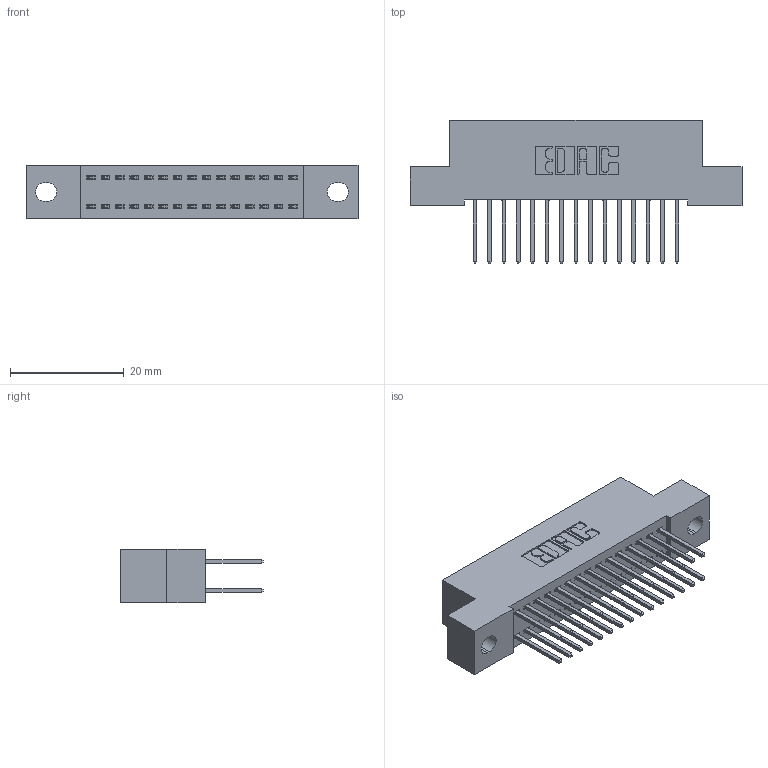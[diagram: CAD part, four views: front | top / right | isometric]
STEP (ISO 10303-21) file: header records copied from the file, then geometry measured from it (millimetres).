
FILE_DESCRIPTION (( 'STEP AP203' ), '1' );
FILE_NAME ('392-030-523-202.STEP', '2018-08-15T22:16:20', ( '' ), ( '' ), 'SwSTEP 2.0', 'SolidWorks 2016', '' );
FILE_SCHEMA (( 'CONFIG_CONTROL_DESIGN' ));
Length unit declared in the file: inch
Products named in the file (3): 342 Part_.128 Slot; 345-292-001_345-293-123; 392-030-523-202
Assembly tree (31 placements, depth 2):
  392-030-523-202
    342 Part_.128 Slot
    345-292-001_345-293-123  x30
Bounding box: 58.42 x 25.15 x 9.4 mm (x, y, z)
Volume: 5130.6 mm3; surface area: 7707.1 mm2
Topology: 31 solids, 31 shells, 1674 faces, 4961 edges, 3266 vertices
Faces by surface type: plane 1150, cylinder 524
Entity records: 13163 total; most frequent: CARTESIAN_POINT 2214, ORIENTED_EDGE 2150, DIRECTION 1939, EDGE_CURVE 1075, LINE 947, VECTOR 947, VERTEX_POINT 714, AXIS2_PLACEMENT_3D 496
